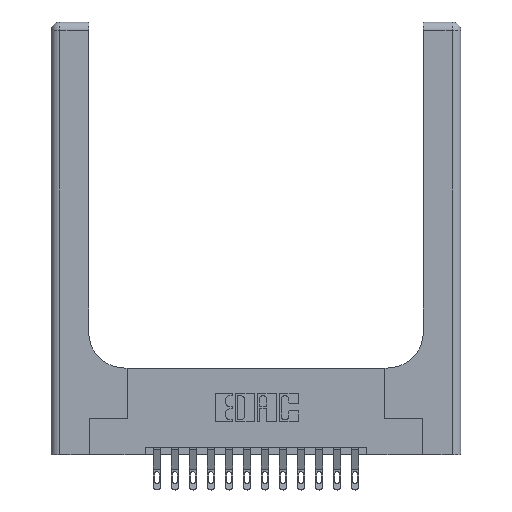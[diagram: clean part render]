
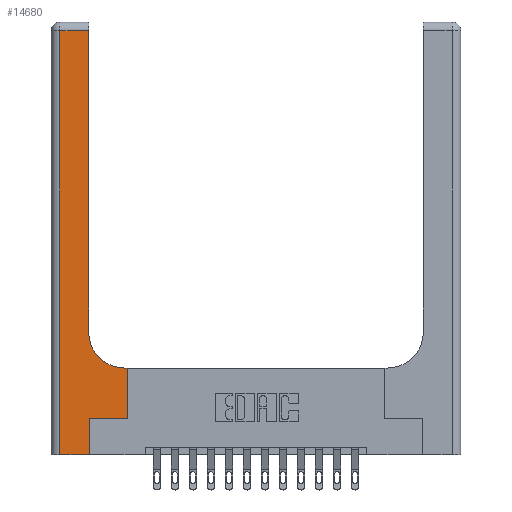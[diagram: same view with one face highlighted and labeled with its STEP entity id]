
A CAD part, top view. The second image highlights one B-rep face of the part: STEP entity #14680.
In plain terms, the highlighted planar face has unit normal (0, 0, 1).
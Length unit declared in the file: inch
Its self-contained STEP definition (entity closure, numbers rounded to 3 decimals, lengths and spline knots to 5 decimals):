
#180 = DIRECTION ( 'NONE',  ( 1., 0., 0. ) ) ;
#284 = CARTESIAN_POINT ( 'NONE',  ( 0.528, 0.25, 0.37 ) ) ;
#313 = DIRECTION ( 'NONE',  ( 0., 0., -1. ) ) ;
#946 = ORIENTED_EDGE ( 'NONE', *, *, #9416, .T. ) ;
#1412 = VERTEX_POINT ( 'NONE', #8186 ) ;
#1532 = LINE ( 'NONE', #16505, #16317 ) ;
#2166 = VECTOR ( 'NONE', #4364, 39.37008 ) ;
#2312 = LINE ( 'NONE', #6385, #15430 ) ;
#2436 = CARTESIAN_POINT ( 'NONE',  ( 0.51, 0.6, 0.37 ) ) ;
#2553 = LINE ( 'NONE', #9322, #6113 ) ;
#2746 = ORIENTED_EDGE ( 'NONE', *, *, #9785, .T. ) ;
#2857 = VERTEX_POINT ( 'NONE', #15106 ) ;
#3078 = VECTOR ( 'NONE', #180, 39.37008 ) ;
#3182 = EDGE_CURVE ( 'NONE', #3821, #1412, #2553, .T. ) ;
#3202 = PLANE ( 'NONE',  #15684 ) ;
#3814 = CARTESIAN_POINT ( 'NONE',  ( 0.265, 0., 0.37 ) ) ;
#3821 = VERTEX_POINT ( 'NONE', #8361 ) ;
#3926 = VERTEX_POINT ( 'NONE', #12590 ) ;
#4364 = DIRECTION ( 'NONE',  ( 1., 0., 0. ) ) ;
#4458 = LINE ( 'NONE', #16788, #2166 ) ;
#4915 = DIRECTION ( 'NONE',  ( 0., 1., 0. ) ) ;
#5428 = LINE ( 'NONE', #14973, #3078 ) ;
#5698 = CARTESIAN_POINT ( 'NONE',  ( 0.51, 0.85, 0.37 ) ) ;
#5777 = CIRCLE ( 'NONE', #17283, 0.25 ) ;
#6113 = VECTOR ( 'NONE', #6618, 39.37008 ) ;
#6319 = EDGE_CURVE ( 'NONE', #9218, #10714, #16248, .T. ) ;
#6385 = CARTESIAN_POINT ( 'NONE',  ( 0., 2.94, 0.37 ) ) ;
#6495 = CARTESIAN_POINT ( 'NONE',  ( 0.26, 0.85, 0.37 ) ) ;
#6618 = DIRECTION ( 'NONE',  ( 0., -1., 0. ) ) ;
#6696 = DIRECTION ( 'NONE',  ( 0., 1., 0. ) ) ;
#7244 = ORIENTED_EDGE ( 'NONE', *, *, #3182, .T. ) ;
#7523 = DIRECTION ( 'NONE',  ( 0., 1., 0. ) ) ;
#7820 = DIRECTION ( 'NONE',  ( -1., 0., 0. ) ) ;
#8186 = CARTESIAN_POINT ( 'NONE',  ( 0.06, 0., 0.37 ) ) ;
#8199 = ORIENTED_EDGE ( 'NONE', *, *, #15657, .T. ) ;
#8361 = CARTESIAN_POINT ( 'NONE',  ( 0.06, 2.94, 0.37 ) ) ;
#8686 = DIRECTION ( 'NONE',  ( -1., 0., 0. ) ) ;
#8949 = CARTESIAN_POINT ( 'NONE',  ( 0.265, 0.25, 0.37 ) ) ;
#9218 = VERTEX_POINT ( 'NONE', #15000 ) ;
#9322 = CARTESIAN_POINT ( 'NONE',  ( 0.06, 3., 0.37 ) ) ;
#9333 = ORIENTED_EDGE ( 'NONE', *, *, #15166, .T. ) ;
#9416 = EDGE_CURVE ( 'NONE', #11028, #2857, #15624, .T. ) ;
#9785 = EDGE_CURVE ( 'NONE', #13592, #9980, #5777, .T. ) ;
#9980 = VERTEX_POINT ( 'NONE', #6495 ) ;
#10079 = ORIENTED_EDGE ( 'NONE', *, *, #16485, .T. ) ;
#10661 = CARTESIAN_POINT ( 'NONE',  ( 0.26, 3., 0.37 ) ) ;
#10714 = VERTEX_POINT ( 'NONE', #8949 ) ;
#10721 = ORIENTED_EDGE ( 'NONE', *, *, #16605, .T. ) ;
#10800 = EDGE_LOOP ( 'NONE', ( #16966, #8199, #7244, #10721, #12732, #9333, #946, #10079, #2746 ) ) ;
#11028 = VERTEX_POINT ( 'NONE', #284 ) ;
#11194 = DIRECTION ( 'NONE',  ( 0., 0., -1. ) ) ;
#12590 = CARTESIAN_POINT ( 'NONE',  ( 0.26, 2.94, 0.37 ) ) ;
#12732 = ORIENTED_EDGE ( 'NONE', *, *, #6319, .T. ) ;
#12918 = CARTESIAN_POINT ( 'NONE',  ( 0., 3., 0.37 ) ) ;
#13592 = VERTEX_POINT ( 'NONE', #2436 ) ;
#13608 = DIRECTION ( 'NONE',  ( -1., 0., 0. ) ) ;
#14260 = VECTOR ( 'NONE', #4915, 39.37008 ) ;
#14620 = CARTESIAN_POINT ( 'NONE',  ( 0.528, 0.25, 0.37 ) ) ;
#14635 = LINE ( 'NONE', #10661, #14260 ) ;
#14680 = ADVANCED_FACE ( 'NONE', ( #15636 ), #3202, .F. ) ;
#14838 = EDGE_CURVE ( 'NONE', #9980, #3926, #14635, .T. ) ;
#14973 = CARTESIAN_POINT ( 'NONE',  ( 0., 0., 0.37 ) ) ;
#15000 = CARTESIAN_POINT ( 'NONE',  ( 0.265, 0., 0.37 ) ) ;
#15106 = CARTESIAN_POINT ( 'NONE',  ( 0.528, 0.6, 0.37 ) ) ;
#15166 = EDGE_CURVE ( 'NONE', #10714, #11028, #4458, .T. ) ;
#15430 = VECTOR ( 'NONE', #7820, 39.37008 ) ;
#15624 = LINE ( 'NONE', #14620, #17522 ) ;
#15636 = FACE_OUTER_BOUND ( 'NONE', #10800, .T. ) ;
#15657 = EDGE_CURVE ( 'NONE', #3926, #3821, #2312, .T. ) ;
#15684 = AXIS2_PLACEMENT_3D ( 'NONE', #12918, #313, #8686 ) ;
#15838 = VECTOR ( 'NONE', #6696, 39.37008 ) ;
#16248 = LINE ( 'NONE', #3814, #15838 ) ;
#16317 = VECTOR ( 'NONE', #13608, 39.37008 ) ;
#16485 = EDGE_CURVE ( 'NONE', #2857, #13592, #1532, .T. ) ;
#16505 = CARTESIAN_POINT ( 'NONE',  ( 0.26, 0.6, 0.37 ) ) ;
#16605 = EDGE_CURVE ( 'NONE', #1412, #9218, #5428, .T. ) ;
#16689 = DIRECTION ( 'NONE',  ( 1., 0., 0. ) ) ;
#16788 = CARTESIAN_POINT ( 'NONE',  ( 0.265, 0.25, 0.37 ) ) ;
#16966 = ORIENTED_EDGE ( 'NONE', *, *, #14838, .T. ) ;
#17283 = AXIS2_PLACEMENT_3D ( 'NONE', #5698, #11194, #16689 ) ;
#17522 = VECTOR ( 'NONE', #7523, 39.37008 ) ;
